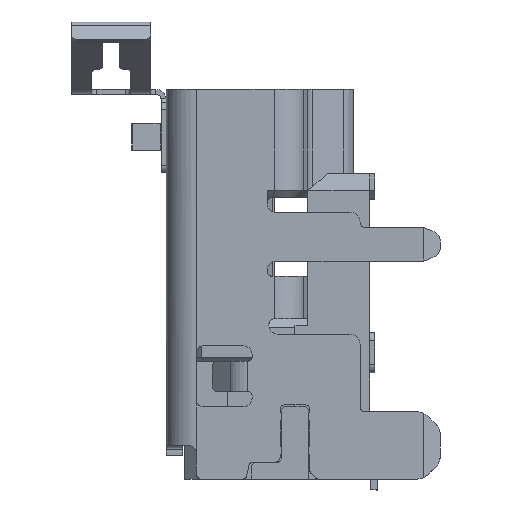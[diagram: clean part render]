
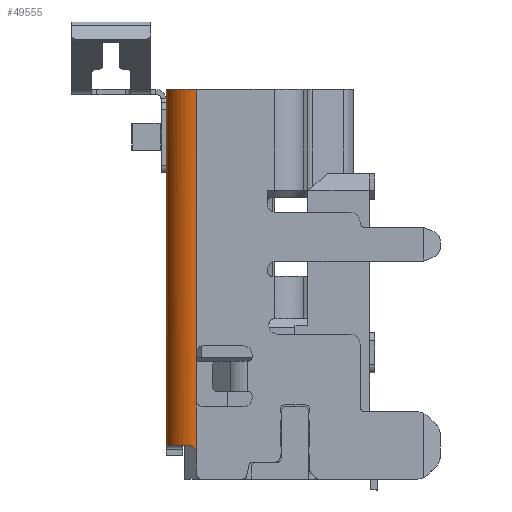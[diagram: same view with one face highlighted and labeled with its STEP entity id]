
A CAD part, left-side view. The second image highlights one B-rep face of the part: STEP entity #49555.
In plain terms, the highlighted cylindrical face has radius 0.9 mm (diameter 1.8 mm), a partial arc.
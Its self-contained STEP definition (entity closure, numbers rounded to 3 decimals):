
#3646 = EDGE_LOOP ( 'NONE', ( #46353, #76094, #109982, #44853, #72048, #96266, #63590 ) ) ;
#5767 = DIRECTION ( 'NONE',  ( 0., 0., 1. ) ) ;
#8880 = VERTEX_POINT ( 'NONE', #14715 ) ;
#12114 = DIRECTION ( 'NONE',  ( 0., 0., 1. ) ) ;
#14715 = CARTESIAN_POINT ( 'NONE',  ( -7.5, -0.375, -8.3 ) ) ;
#18248 = CARTESIAN_POINT ( 'NONE',  ( -7.493, -0.254, -8.076 ) ) ;
#18825 = CARTESIAN_POINT ( 'NONE',  ( -7.5, -0.375, -8.3 ) ) ;
#19453 = VERTEX_POINT ( 'NONE', #103069 ) ;
#19586 = AXIS2_PLACEMENT_3D ( 'NONE', #102678, #40136, #77048 ) ;
#19780 = EDGE_CURVE ( 'NONE', #95696, #8880, #80021, .T. ) ;
#19902 = CARTESIAN_POINT ( 'NONE',  ( -6.6, -0.375, -8.365 ) ) ;
#21648 = DIRECTION ( 'NONE',  ( 1., 0., 0. ) ) ;
#27149 = CARTESIAN_POINT ( 'NONE',  ( -6.6, 0.525, 2.5 ) ) ;
#28039 = DIRECTION ( 'NONE',  ( 1., 0., 0. ) ) ;
#32330 = EDGE_CURVE ( 'NONE', #67311, #64069, #116000, .T. ) ;
#36158 = EDGE_CURVE ( 'NONE', #64069, #70389, #48199, .T. ) ;
#40136 = DIRECTION ( 'NONE',  ( 0., 0., 1. ) ) ;
#44853 = ORIENTED_EDGE ( 'NONE', *, *, #56917, .T. ) ;
#46353 = ORIENTED_EDGE ( 'NONE', *, *, #32330, .F. ) ;
#47329 = CYLINDRICAL_SURFACE ( 'NONE', #61441, 0.9 ) ;
#48199 = CIRCLE ( 'NONE', #19586, 0.9 ) ;
#49555 = ADVANCED_FACE ( 'NONE', ( #75288 ), #47329, .T. ) ;
#50974 = CARTESIAN_POINT ( 'NONE',  ( -7.5, -0.375, -6.7 ) ) ;
#51156 = CARTESIAN_POINT ( 'NONE',  ( -7.5, -0.375, -8.365 ) ) ;
#53319 = EDGE_CURVE ( 'NONE', #101817, #19453, #103855, .T. ) ;
#53678 = DIRECTION ( 'NONE',  ( 0., 0., 1. ) ) ;
#56917 = EDGE_CURVE ( 'NONE', #8880, #101817, #116066, .T. ) ;
#59486 = DIRECTION ( 'NONE',  ( 0., 0., 1. ) ) ;
#61441 = AXIS2_PLACEMENT_3D ( 'NONE', #19902, #111639, #21648 ) ;
#63036 = AXIS2_PLACEMENT_3D ( 'NONE', #98942, #53678, #28039 ) ;
#63590 = ORIENTED_EDGE ( 'NONE', *, *, #36158, .F. ) ;
#64069 = VERTEX_POINT ( 'NONE', #27149 ) ;
#64891 = EDGE_CURVE ( 'NONE', #67311, #95696, #85926, .T. ) ;
#65764 = CARTESIAN_POINT ( 'NONE',  ( -7.5, -0.375, -8.365 ) ) ;
#67311 = VERTEX_POINT ( 'NONE', #115248 ) ;
#70389 = VERTEX_POINT ( 'NONE', #114175 ) ;
#72048 = ORIENTED_EDGE ( 'NONE', *, *, #53319, .T. ) ;
#73632 = CARTESIAN_POINT ( 'NONE',  ( -7.465, -0.125, -8.05 ) ) ;
#75288 = FACE_OUTER_BOUND ( 'NONE', #3646, .T. ) ;
#76094 = ORIENTED_EDGE ( 'NONE', *, *, #64891, .T. ) ;
#76542 = CARTESIAN_POINT ( 'NONE',  ( -7.5, -0.375, -8.365 ) ) ;
#77048 = DIRECTION ( 'NONE',  ( 1., 0., 0. ) ) ;
#77273 = VECTOR ( 'NONE', #59486, 1000. ) ;
#80021 = B_SPLINE_CURVE_WITH_KNOTS ( 'NONE', 3,
 ( #73632, #99856, #18248, #83771, #108803, #18825 ),
 .UNSPECIFIED., .F., .F.,
 ( 4, 2, 4 ),
 ( 0., 0.5, 1. ),
 .UNSPECIFIED. ) ;
#83771 = CARTESIAN_POINT ( 'NONE',  ( -7.501, -0.347, -8.168 ) ) ;
#84399 = EDGE_CURVE ( 'NONE', #19453, #70389, #105121, .T. ) ;
#85926 = CIRCLE ( 'NONE', #63036, 0.9 ) ;
#88840 = VECTOR ( 'NONE', #95001, 1000. ) ;
#89610 = VECTOR ( 'NONE', #5767, 1000. ) ;
#93040 = CARTESIAN_POINT ( 'NONE',  ( -7.465, -0.125, -8.05 ) ) ;
#95001 = DIRECTION ( 'NONE',  ( 0., 0., 1. ) ) ;
#95696 = VERTEX_POINT ( 'NONE', #93040 ) ;
#96266 = ORIENTED_EDGE ( 'NONE', *, *, #84399, .T. ) ;
#98942 = CARTESIAN_POINT ( 'NONE',  ( -6.6, -0.375, -8.05 ) ) ;
#99856 = CARTESIAN_POINT ( 'NONE',  ( -7.483, -0.189, -8.05 ) ) ;
#101817 = VERTEX_POINT ( 'NONE', #50974 ) ;
#102678 = CARTESIAN_POINT ( 'NONE',  ( -6.6, -0.375, 2.5 ) ) ;
#103069 = CARTESIAN_POINT ( 'NONE',  ( -7.5, -0.375, -5.3 ) ) ;
#103855 = LINE ( 'NONE', #65764, #113579 ) ;
#105121 = LINE ( 'NONE', #76542, #88840 ) ;
#107044 = CARTESIAN_POINT ( 'NONE',  ( -6.6, 0.525, 2.5 ) ) ;
#108803 = CARTESIAN_POINT ( 'NONE',  ( -7.5, -0.375, -8.233 ) ) ;
#109982 = ORIENTED_EDGE ( 'NONE', *, *, #19780, .T. ) ;
#111639 = DIRECTION ( 'NONE',  ( 0., 0., 1. ) ) ;
#113579 = VECTOR ( 'NONE', #12114, 1000. ) ;
#114175 = CARTESIAN_POINT ( 'NONE',  ( -7.5, -0.375, 2.5 ) ) ;
#115248 = CARTESIAN_POINT ( 'NONE',  ( -6.6, 0.525, -8.05 ) ) ;
#116000 = LINE ( 'NONE', #107044, #89610 ) ;
#116066 = LINE ( 'NONE', #51156, #77273 ) ;
